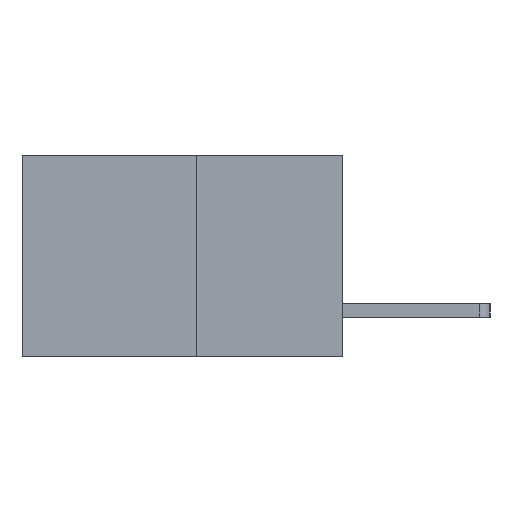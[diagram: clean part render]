
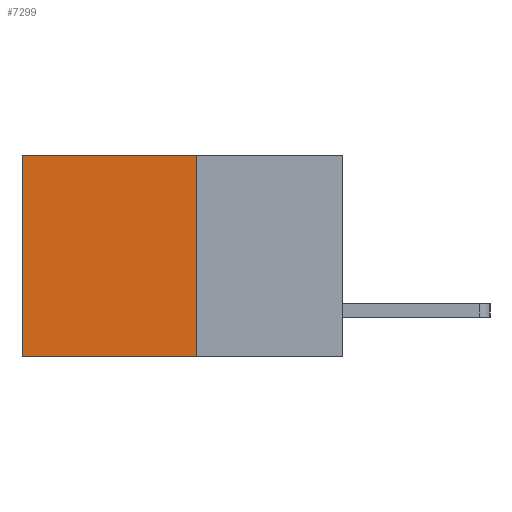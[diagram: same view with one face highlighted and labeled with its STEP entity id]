
A CAD part, left-side view. The second image highlights one B-rep face of the part: STEP entity #7299.
In plain terms, the highlighted planar face has unit normal (-1, 0, 0).
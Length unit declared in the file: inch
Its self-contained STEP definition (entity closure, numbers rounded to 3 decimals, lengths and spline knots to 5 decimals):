
#6 = AXIS2_PLACEMENT_3D ( 'NONE', #7889, #7871, #7859 ) ;
#686 = CARTESIAN_POINT ( 'NONE',  ( 0.277, 0.59, 0. ) ) ;
#776 = EDGE_CURVE ( 'NONE', #3355, #5910, #4326, .T. ) ;
#1469 = VERTEX_POINT ( 'NONE', #686 ) ;
#1961 = VECTOR ( 'NONE', #4470, 39.37008 ) ;
#2488 = ORIENTED_EDGE ( 'NONE', *, *, #2974, .T. ) ;
#2515 = VECTOR ( 'NONE', #6731, 39.37008 ) ;
#2719 = EDGE_LOOP ( 'NONE', ( #4416, #2892, #4388, #2488 ) ) ;
#2892 = ORIENTED_EDGE ( 'NONE', *, *, #776, .F. ) ;
#2974 = EDGE_CURVE ( 'NONE', #5280, #1469, #7809, .T. ) ;
#3355 = VERTEX_POINT ( 'NONE', #6774 ) ;
#3522 = FACE_OUTER_BOUND ( 'NONE', #2719, .T. ) ;
#3757 = LINE ( 'NONE', #4453, #1961 ) ;
#4060 = DIRECTION ( 'NONE',  ( 0., 1., 0. ) ) ;
#4223 = CARTESIAN_POINT ( 'NONE',  ( 0.277, 0.27, 0. ) ) ;
#4326 = LINE ( 'NONE', #7345, #2515 ) ;
#4388 = ORIENTED_EDGE ( 'NONE', *, *, #6841, .F. ) ;
#4416 = ORIENTED_EDGE ( 'NONE', *, *, #7673, .T. ) ;
#4453 = CARTESIAN_POINT ( 'NONE',  ( 0.277, 0.27, -0.37 ) ) ;
#4470 = DIRECTION ( 'NONE',  ( 0., 0., -1. ) ) ;
#4598 = VECTOR ( 'NONE', #5906, 39.37008 ) ;
#5280 = VERTEX_POINT ( 'NONE', #7099 ) ;
#5830 = CARTESIAN_POINT ( 'NONE',  ( 0.277, 0.59, -0.37 ) ) ;
#5906 = DIRECTION ( 'NONE',  ( 0., 0., -1. ) ) ;
#5910 = VERTEX_POINT ( 'NONE', #5830 ) ;
#5943 = CARTESIAN_POINT ( 'NONE',  ( 0.277, 0.59, -0.37 ) ) ;
#6064 = VECTOR ( 'NONE', #4060, 39.37008 ) ;
#6157 = LINE ( 'NONE', #5943, #4598 ) ;
#6731 = DIRECTION ( 'NONE',  ( 0., 1., 0. ) ) ;
#6774 = CARTESIAN_POINT ( 'NONE',  ( 0.277, 0.27, -0.37 ) ) ;
#6841 = EDGE_CURVE ( 'NONE', #5280, #3355, #3757, .T. ) ;
#7099 = CARTESIAN_POINT ( 'NONE',  ( 0.277, 0.27, 0. ) ) ;
#7299 = ADVANCED_FACE ( 'NONE', ( #3522 ), #7910, .F. ) ;
#7345 = CARTESIAN_POINT ( 'NONE',  ( 0.277, 0.27, -0.37 ) ) ;
#7673 = EDGE_CURVE ( 'NONE', #1469, #5910, #6157, .T. ) ;
#7809 = LINE ( 'NONE', #4223, #6064 ) ;
#7859 = DIRECTION ( 'NONE',  ( 0., 0., -1. ) ) ;
#7871 = DIRECTION ( 'NONE',  ( 1., 0., 0. ) ) ;
#7889 = CARTESIAN_POINT ( 'NONE',  ( 0.277, 0.27, -0.37 ) ) ;
#7910 = PLANE ( 'NONE',  #6 ) ;
